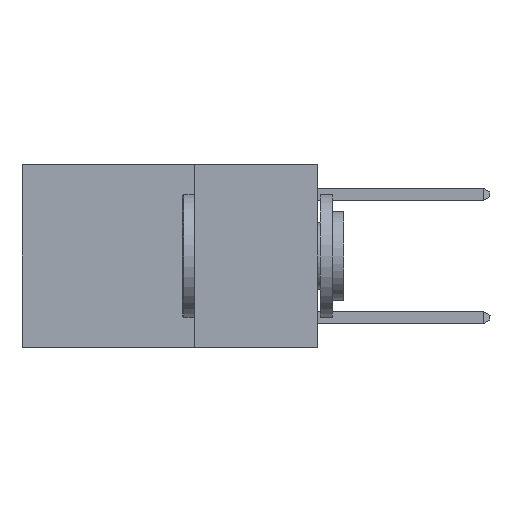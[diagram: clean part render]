
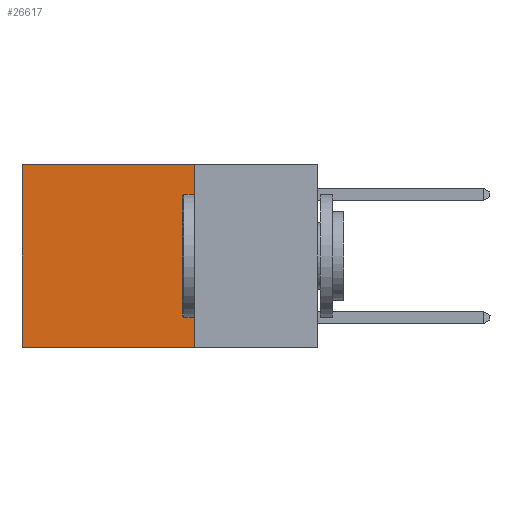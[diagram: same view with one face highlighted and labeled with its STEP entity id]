
A CAD part, left-side view. The second image highlights one B-rep face of the part: STEP entity #26617.
In plain terms, the highlighted planar face has unit normal (-1, 0, 0).
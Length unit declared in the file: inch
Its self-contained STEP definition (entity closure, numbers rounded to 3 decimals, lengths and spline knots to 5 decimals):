
#107 = DIRECTION ( 'NONE',  ( 0., 0., -1. ) ) ;
#991 = CARTESIAN_POINT ( 'NONE',  ( 0.2625, 0.25, -0.37 ) ) ;
#1745 = CARTESIAN_POINT ( 'NONE',  ( 0.2625, 0.25, -0.37 ) ) ;
#2194 = PLANE ( 'NONE',  #23427 ) ;
#2877 = LINE ( 'NONE', #23722, #7573 ) ;
#3434 = VECTOR ( 'NONE', #7314, 39.37008 ) ;
#3444 = EDGE_CURVE ( 'NONE', #17318, #4883, #14119, .T. ) ;
#4422 = VECTOR ( 'NONE', #107, 39.37008 ) ;
#4883 = VERTEX_POINT ( 'NONE', #11965 ) ;
#5052 = CARTESIAN_POINT ( 'NONE',  ( 0.2625, 0.6, 0. ) ) ;
#5516 = VERTEX_POINT ( 'NONE', #22544 ) ;
#5974 = EDGE_CURVE ( 'NONE', #7201, #17318, #10784, .T. ) ;
#6089 = EDGE_CURVE ( 'NONE', #5516, #4883, #9111, .T. ) ;
#7201 = VERTEX_POINT ( 'NONE', #17316 ) ;
#7314 = DIRECTION ( 'NONE',  ( 0., 0., -1. ) ) ;
#7573 = VECTOR ( 'NONE', #12733, 39.37008 ) ;
#7980 = ORIENTED_EDGE ( 'NONE', *, *, #3444, .F. ) ;
#8454 = CARTESIAN_POINT ( 'NONE',  ( 0.2625, 0.25, 0. ) ) ;
#9111 = LINE ( 'NONE', #5052, #3434 ) ;
#10658 = ORIENTED_EDGE ( 'NONE', *, *, #21624, .T. ) ;
#10784 = LINE ( 'NONE', #21676, #4422 ) ;
#11614 = ORIENTED_EDGE ( 'NONE', *, *, #6089, .T. ) ;
#11965 = CARTESIAN_POINT ( 'NONE',  ( 0.2625, 0.6, -0.37 ) ) ;
#12733 = DIRECTION ( 'NONE',  ( 0., 1., 0. ) ) ;
#13899 = ORIENTED_EDGE ( 'NONE', *, *, #5974, .F. ) ;
#14119 = LINE ( 'NONE', #1745, #26759 ) ;
#16852 = DIRECTION ( 'NONE',  ( 0., 1., 0. ) ) ;
#17316 = CARTESIAN_POINT ( 'NONE',  ( 0.2625, 0.25, 0. ) ) ;
#17318 = VERTEX_POINT ( 'NONE', #991 ) ;
#21221 = FACE_OUTER_BOUND ( 'NONE', #21568, .T. ) ;
#21431 = DIRECTION ( 'NONE',  ( 1., 0., 0. ) ) ;
#21568 = EDGE_LOOP ( 'NONE', ( #11614, #7980, #13899, #10658 ) ) ;
#21624 = EDGE_CURVE ( 'NONE', #7201, #5516, #2877, .T. ) ;
#21676 = CARTESIAN_POINT ( 'NONE',  ( 0.2625, 0.25, 0. ) ) ;
#22544 = CARTESIAN_POINT ( 'NONE',  ( 0.2625, 0.6, 0. ) ) ;
#23392 = DIRECTION ( 'NONE',  ( 0., 0., -1. ) ) ;
#23427 = AXIS2_PLACEMENT_3D ( 'NONE', #8454, #21431, #23392 ) ;
#23722 = CARTESIAN_POINT ( 'NONE',  ( 0.2625, 0.25, 0. ) ) ;
#26617 = ADVANCED_FACE ( 'NONE', ( #21221 ), #2194, .F. ) ;
#26759 = VECTOR ( 'NONE', #16852, 39.37008 ) ;
